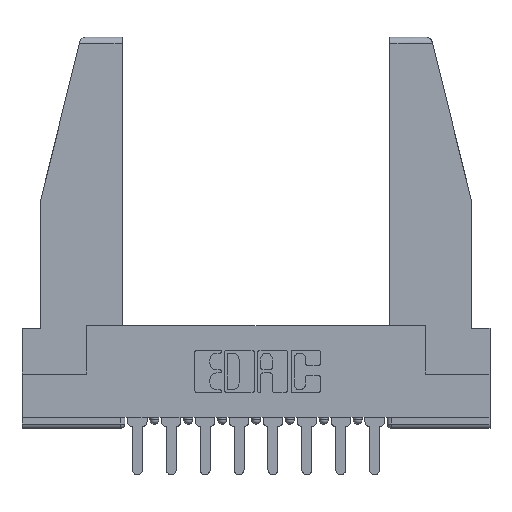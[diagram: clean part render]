
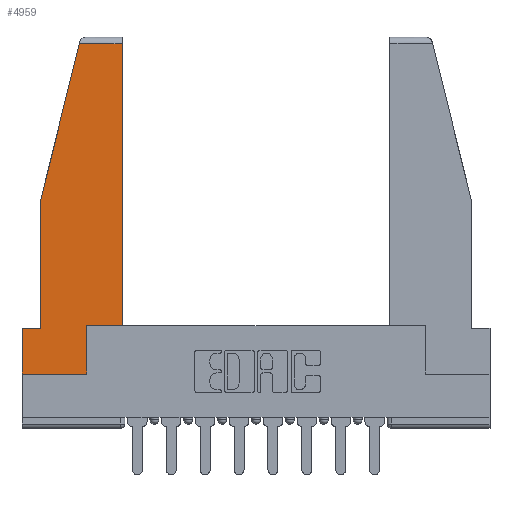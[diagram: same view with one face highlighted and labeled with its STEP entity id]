
A CAD part, top view. The second image highlights one B-rep face of the part: STEP entity #4959.
In plain terms, the highlighted planar face has unit normal (0, 0, 1).
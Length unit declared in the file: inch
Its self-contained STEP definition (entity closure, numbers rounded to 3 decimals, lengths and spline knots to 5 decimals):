
#42 = DIRECTION ( 'NONE',  ( -0.239, -0.971, 0. ) ) ;
#131 = AXIS2_PLACEMENT_3D ( 'NONE', #11985, #6655, #1499 ) ;
#249 = VECTOR ( 'NONE', #4040, 39.37008 ) ;
#1062 = LINE ( 'NONE', #5011, #249 ) ;
#1095 = LINE ( 'NONE', #9146, #11815 ) ;
#1115 = DIRECTION ( 'NONE',  ( 0., 1., 0. ) ) ;
#1295 = CARTESIAN_POINT ( 'NONE',  ( 0., 0., 0. ) ) ;
#1298 = VECTOR ( 'NONE', #1115, 39.37008 ) ;
#1499 = DIRECTION ( 'NONE',  ( 1., 0., 0. ) ) ;
#1526 = CARTESIAN_POINT ( 'NONE',  ( 0., 1.52, 0. ) ) ;
#1863 = CARTESIAN_POINT ( 'NONE',  ( 0.461, 0.223, 0. ) ) ;
#1908 = VERTEX_POINT ( 'NONE', #8970 ) ;
#2187 = DIRECTION ( 'NONE',  ( 0., -1., 0. ) ) ;
#2216 = LINE ( 'NONE', #7400, #6302 ) ;
#2833 = VECTOR ( 'NONE', #11506, 39.37008 ) ;
#2896 = DIRECTION ( 'NONE',  ( 0., -1., 0. ) ) ;
#3094 = ORIENTED_EDGE ( 'NONE', *, *, #8637, .T. ) ;
#3477 = CARTESIAN_POINT ( 'NONE',  ( 0.297, 0., 0. ) ) ;
#3677 = EDGE_CURVE ( 'NONE', #10622, #5987, #1095, .T. ) ;
#3943 = VECTOR ( 'NONE', #6674, 39.37008 ) ;
#4040 = DIRECTION ( 'NONE',  ( 1., 0., 0. ) ) ;
#4130 = ORIENTED_EDGE ( 'NONE', *, *, #3677, .T. ) ;
#4172 = CARTESIAN_POINT ( 'NONE',  ( 0.271, 1.55, 0. ) ) ;
#4443 = LINE ( 'NONE', #6311, #2833 ) ;
#4633 = LINE ( 'NONE', #5367, #12925 ) ;
#4654 = DIRECTION ( 'NONE',  ( -1., 0., 0. ) ) ;
#4803 = CARTESIAN_POINT ( 'NONE',  ( 0.2636, 1.52, 0. ) ) ;
#4823 = EDGE_CURVE ( 'NONE', #10940, #11245, #4443, .T. ) ;
#4959 = ADVANCED_FACE ( 'NONE', ( #12074 ), #5472, .T. ) ;
#5011 = CARTESIAN_POINT ( 'NONE',  ( 0., 0., 0. ) ) ;
#5110 = ORIENTED_EDGE ( 'NONE', *, *, #8409, .T. ) ;
#5232 = CARTESIAN_POINT ( 'NONE',  ( 0.297, 0., 0. ) ) ;
#5367 = CARTESIAN_POINT ( 'NONE',  ( 0.086, 0.8, 0. ) ) ;
#5472 = PLANE ( 'NONE',  #131 ) ;
#5669 = VERTEX_POINT ( 'NONE', #8653 ) ;
#5987 = VERTEX_POINT ( 'NONE', #1295 ) ;
#6075 = VERTEX_POINT ( 'NONE', #4803 ) ;
#6302 = VECTOR ( 'NONE', #4654, 39.37008 ) ;
#6311 = CARTESIAN_POINT ( 'NONE',  ( 0.461, 0.223, 0. ) ) ;
#6436 = ORIENTED_EDGE ( 'NONE', *, *, #9386, .T. ) ;
#6655 = DIRECTION ( 'NONE',  ( 0., 0., 1. ) ) ;
#6674 = DIRECTION ( 'NONE',  ( -1., 0., 0. ) ) ;
#6857 = LINE ( 'NONE', #5232, #1298 ) ;
#7400 = CARTESIAN_POINT ( 'NONE',  ( 0., 0.21, 0. ) ) ;
#7594 = ORIENTED_EDGE ( 'NONE', *, *, #8656, .T. ) ;
#7609 = CARTESIAN_POINT ( 'NONE',  ( 0., 0.21, 0. ) ) ;
#7657 = EDGE_CURVE ( 'NONE', #5669, #10622, #2216, .T. ) ;
#8402 = LINE ( 'NONE', #4172, #13266 ) ;
#8409 = EDGE_CURVE ( 'NONE', #11605, #10940, #8720, .T. ) ;
#8462 = EDGE_CURVE ( 'NONE', #5987, #8911, #1062, .T. ) ;
#8637 = EDGE_CURVE ( 'NONE', #6075, #1908, #8402, .T. ) ;
#8653 = CARTESIAN_POINT ( 'NONE',  ( 0.086, 0.21, 0. ) ) ;
#8656 = EDGE_CURVE ( 'NONE', #1908, #5669, #4633, .T. ) ;
#8694 = LINE ( 'NONE', #1526, #3943 ) ;
#8720 = LINE ( 'NONE', #8983, #10179 ) ;
#8810 = CARTESIAN_POINT ( 'NONE',  ( 0.461, 1.52, 0. ) ) ;
#8911 = VERTEX_POINT ( 'NONE', #3477 ) ;
#8970 = CARTESIAN_POINT ( 'NONE',  ( 0.086, 0.8, 0. ) ) ;
#8983 = CARTESIAN_POINT ( 'NONE',  ( 0.297, 0.223, 0. ) ) ;
#9146 = CARTESIAN_POINT ( 'NONE',  ( 0., 0.21, 0. ) ) ;
#9386 = EDGE_CURVE ( 'NONE', #11245, #6075, #8694, .T. ) ;
#10179 = VECTOR ( 'NONE', #11002, 39.37008 ) ;
#10622 = VERTEX_POINT ( 'NONE', #7609 ) ;
#10916 = ORIENTED_EDGE ( 'NONE', *, *, #11080, .T. ) ;
#10940 = VERTEX_POINT ( 'NONE', #1863 ) ;
#11002 = DIRECTION ( 'NONE',  ( 1., 0., 0. ) ) ;
#11080 = EDGE_CURVE ( 'NONE', #8911, #11605, #6857, .T. ) ;
#11231 = ORIENTED_EDGE ( 'NONE', *, *, #4823, .T. ) ;
#11245 = VERTEX_POINT ( 'NONE', #8810 ) ;
#11475 = CARTESIAN_POINT ( 'NONE',  ( 0.297, 0.223, 0. ) ) ;
#11506 = DIRECTION ( 'NONE',  ( 0., 1., 0. ) ) ;
#11605 = VERTEX_POINT ( 'NONE', #11475 ) ;
#11619 = EDGE_LOOP ( 'NONE', ( #11231, #6436, #3094, #7594, #11971, #4130, #12699, #10916, #5110 ) ) ;
#11815 = VECTOR ( 'NONE', #2896, 39.37008 ) ;
#11971 = ORIENTED_EDGE ( 'NONE', *, *, #7657, .T. ) ;
#11985 = CARTESIAN_POINT ( 'NONE',  ( 0., 0., 0. ) ) ;
#12074 = FACE_OUTER_BOUND ( 'NONE', #11619, .T. ) ;
#12699 = ORIENTED_EDGE ( 'NONE', *, *, #8462, .T. ) ;
#12925 = VECTOR ( 'NONE', #2187, 39.37008 ) ;
#13266 = VECTOR ( 'NONE', #42, 39.37008 ) ;
